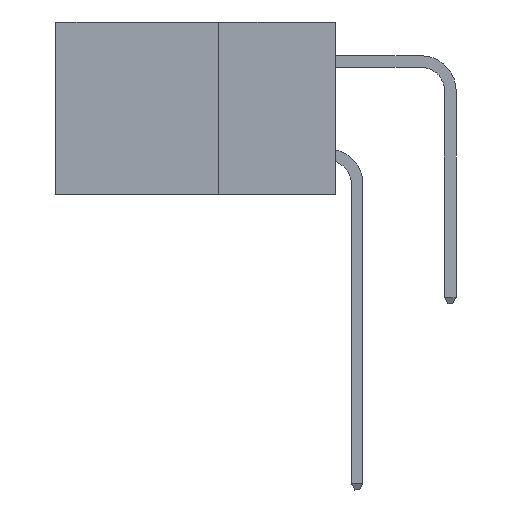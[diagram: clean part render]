
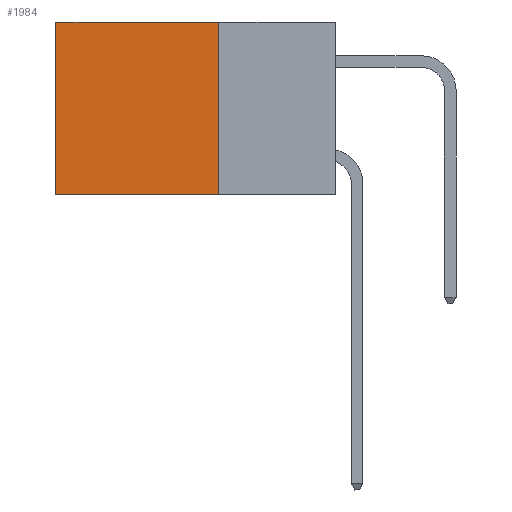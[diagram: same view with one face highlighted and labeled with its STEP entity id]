
A CAD part, left-side view. The second image highlights one B-rep face of the part: STEP entity #1984.
In plain terms, the highlighted planar face has unit normal (-1, 0, 0).
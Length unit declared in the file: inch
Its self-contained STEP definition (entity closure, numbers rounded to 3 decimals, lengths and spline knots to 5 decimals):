
#706 = VECTOR ( 'NONE', #6420, 39.37008 ) ;
#1046 = EDGE_CURVE ( 'NONE', #7055, #21166, #13526, .T. ) ;
#1984 = ADVANCED_FACE ( 'NONE', ( #6123 ), #8341, .F. ) ;
#3116 = LINE ( 'NONE', #24102, #706 ) ;
#3199 = EDGE_CURVE ( 'NONE', #24517, #7055, #7112, .T. ) ;
#3281 = CARTESIAN_POINT ( 'NONE',  ( 0.2875, 0.6, -0.37 ) ) ;
#4349 = VECTOR ( 'NONE', #13797, 39.37008 ) ;
#4543 = CARTESIAN_POINT ( 'NONE',  ( 0.2875, 0.25, -0.37 ) ) ;
#4967 = LINE ( 'NONE', #13224, #28603 ) ;
#5489 = DIRECTION ( 'NONE',  ( 0., 1., 0. ) ) ;
#6123 = FACE_OUTER_BOUND ( 'NONE', #9581, .T. ) ;
#6347 = CARTESIAN_POINT ( 'NONE',  ( 0.2875, 0.6, 0. ) ) ;
#6420 = DIRECTION ( 'NONE',  ( 0., 0., -1. ) ) ;
#6639 = AXIS2_PLACEMENT_3D ( 'NONE', #15356, #13244, #17174 ) ;
#6861 = ORIENTED_EDGE ( 'NONE', *, *, #1046, .F. ) ;
#7055 = VERTEX_POINT ( 'NONE', #4543 ) ;
#7112 = LINE ( 'NONE', #24162, #4349 ) ;
#8341 = PLANE ( 'NONE',  #6639 ) ;
#9010 = VERTEX_POINT ( 'NONE', #6347 ) ;
#9299 = CARTESIAN_POINT ( 'NONE',  ( 0.2875, 0.25, 0. ) ) ;
#9581 = EDGE_LOOP ( 'NONE', ( #11112, #6861, #22478, #16727 ) ) ;
#11112 = ORIENTED_EDGE ( 'NONE', *, *, #14105, .T. ) ;
#12208 = CARTESIAN_POINT ( 'NONE',  ( 0.2875, 0.25, -0.37 ) ) ;
#13224 = CARTESIAN_POINT ( 'NONE',  ( 0.2875, 0.25, 0. ) ) ;
#13244 = DIRECTION ( 'NONE',  ( 1., 0., 0. ) ) ;
#13526 = LINE ( 'NONE', #12208, #16958 ) ;
#13797 = DIRECTION ( 'NONE',  ( 0., 0., -1. ) ) ;
#14105 = EDGE_CURVE ( 'NONE', #9010, #21166, #3116, .T. ) ;
#15356 = CARTESIAN_POINT ( 'NONE',  ( 0.2875, 0.25, 0. ) ) ;
#16727 = ORIENTED_EDGE ( 'NONE', *, *, #27764, .T. ) ;
#16958 = VECTOR ( 'NONE', #5489, 39.37008 ) ;
#17174 = DIRECTION ( 'NONE',  ( 0., 0., -1. ) ) ;
#21166 = VERTEX_POINT ( 'NONE', #3281 ) ;
#22478 = ORIENTED_EDGE ( 'NONE', *, *, #3199, .F. ) ;
#24102 = CARTESIAN_POINT ( 'NONE',  ( 0.2875, 0.6, 0. ) ) ;
#24162 = CARTESIAN_POINT ( 'NONE',  ( 0.2875, 0.25, 0. ) ) ;
#24445 = DIRECTION ( 'NONE',  ( 0., 1., 0. ) ) ;
#24517 = VERTEX_POINT ( 'NONE', #9299 ) ;
#27764 = EDGE_CURVE ( 'NONE', #24517, #9010, #4967, .T. ) ;
#28603 = VECTOR ( 'NONE', #24445, 39.37008 ) ;
